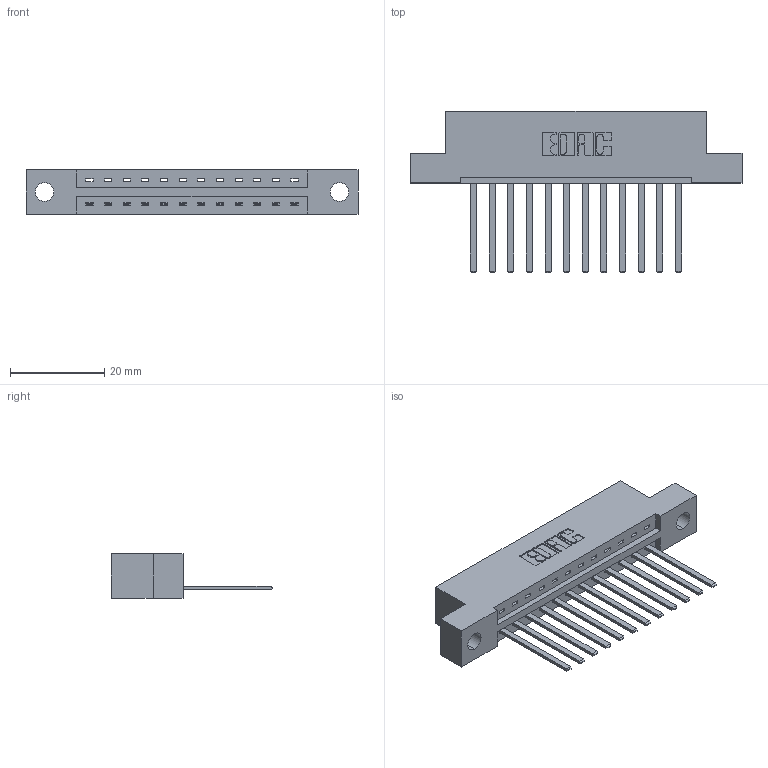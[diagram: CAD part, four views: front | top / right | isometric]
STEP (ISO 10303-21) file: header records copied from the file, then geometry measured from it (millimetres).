
FILE_DESCRIPTION (( 'STEP AP203' ), '1' );
FILE_NAME ('387-012-544-104.STEP', '2019-10-02T13:35:33', ( '' ), ( '' ), 'SwSTEP 2.0', 'SolidWorks 2016', '' );
FILE_SCHEMA (( 'CONFIG_CONTROL_DESIGN' ));
Length unit declared in the file: inch
Products named in the file (3): 387-012-544-104; 345-292-001_345-293-144; 337 Part_Flush Mounting Lugs - 0.156 Dia-TH
Assembly tree (13 placements, depth 2):
  387-012-544-104
    337 Part_Flush Mounting Lugs - 0.156 Dia-TH
    345-292-001_345-293-144  x12
Bounding box: 70.56 x 34.3 x 9.4 mm (x, y, z)
Volume: 7009.4 mm3; surface area: 7329.1 mm2
Topology: 13 solids, 13 shells, 786 faces, 2351 edges, 1550 vertices
Faces by surface type: plane 574, cylinder 212
Entity records: 12619 total; most frequent: CARTESIAN_POINT 2202, ORIENTED_EDGE 2150, DIRECTION 1911, EDGE_CURVE 1075, LINE 951, VECTOR 951, VERTEX_POINT 714, AXIS2_PLACEMENT_3D 480
